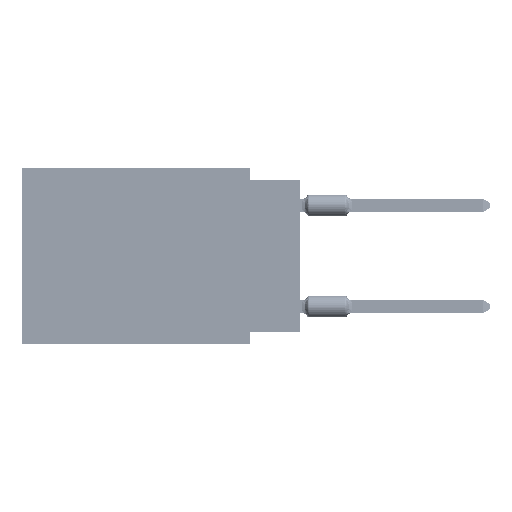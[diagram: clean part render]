
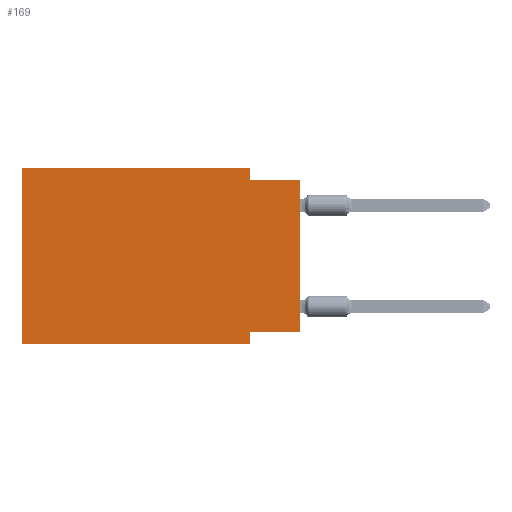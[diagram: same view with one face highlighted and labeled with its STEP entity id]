
A CAD part, left-side view. The second image highlights one B-rep face of the part: STEP entity #169.
In plain terms, the highlighted planar face has unit normal (-1, 0, 0).
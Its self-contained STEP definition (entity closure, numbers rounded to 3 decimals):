
#169 = ADVANCED_FACE ( 'NONE', ( #64927 ), #10518, .F. ) ;
#2532 = LINE ( 'NONE', #24767, #67308 ) ;
#3921 = LINE ( 'NONE', #25838, #35706 ) ;
#4976 = EDGE_CURVE ( 'NONE', #27019, #26516, #2532, .T. ) ;
#5753 = DIRECTION ( 'NONE',  ( 0., 0., -1. ) ) ;
#5892 = VECTOR ( 'NONE', #63146, 1000. ) ;
#6771 = ORIENTED_EDGE ( 'NONE', *, *, #37683, .F. ) ;
#7550 = DIRECTION ( 'NONE',  ( 0., 0., 1. ) ) ;
#10518 = PLANE ( 'NONE',  #65949 ) ;
#13570 = ORIENTED_EDGE ( 'NONE', *, *, #66424, .F. ) ;
#14536 = DIRECTION ( 'NONE',  ( 0., -1., 0. ) ) ;
#15593 = DIRECTION ( 'NONE',  ( 0., 0., -1. ) ) ;
#16460 = EDGE_LOOP ( 'NONE', ( #61674, #40314, #13570, #62673, #17269, #16903, #51655, #6771 ) ) ;
#16903 = ORIENTED_EDGE ( 'NONE', *, *, #4976, .T. ) ;
#17269 = ORIENTED_EDGE ( 'NONE', *, *, #38700, .F. ) ;
#18511 = CARTESIAN_POINT ( 'NONE',  ( 0., 0., -0.635 ) ) ;
#19266 = CARTESIAN_POINT ( 'NONE',  ( 0., 2.54, -8.89 ) ) ;
#19798 = CARTESIAN_POINT ( 'NONE',  ( 0., 13.97, 0. ) ) ;
#20078 = VECTOR ( 'NONE', #61257, 1000. ) ;
#20486 = DIRECTION ( 'NONE',  ( 0., 0., -1. ) ) ;
#23915 = VERTEX_POINT ( 'NONE', #41439 ) ;
#24767 = CARTESIAN_POINT ( 'NONE',  ( 0., 13.97, -8.89 ) ) ;
#25838 = CARTESIAN_POINT ( 'NONE',  ( 0., 2.54, -8.89 ) ) ;
#26011 = LINE ( 'NONE', #65151, #56744 ) ;
#26516 = VERTEX_POINT ( 'NONE', #19266 ) ;
#27019 = VERTEX_POINT ( 'NONE', #66199 ) ;
#29850 = LINE ( 'NONE', #41194, #5892 ) ;
#29943 = VERTEX_POINT ( 'NONE', #40937 ) ;
#30216 = LINE ( 'NONE', #57983, #48218 ) ;
#32770 = CARTESIAN_POINT ( 'NONE',  ( 0., 13.97, 0. ) ) ;
#33168 = VERTEX_POINT ( 'NONE', #66896 ) ;
#35706 = VECTOR ( 'NONE', #15593, 1000. ) ;
#37683 = EDGE_CURVE ( 'NONE', #29943, #44548, #29850, .T. ) ;
#38700 = EDGE_CURVE ( 'NONE', #27019, #33168, #26011, .T. ) ;
#40314 = ORIENTED_EDGE ( 'NONE', *, *, #68638, .F. ) ;
#40388 = EDGE_CURVE ( 'NONE', #44548, #26516, #3921, .T. ) ;
#40937 = CARTESIAN_POINT ( 'NONE',  ( 0., 0., -8.255 ) ) ;
#41194 = CARTESIAN_POINT ( 'NONE',  ( 0., 0., -8.255 ) ) ;
#41439 = CARTESIAN_POINT ( 'NONE',  ( 0., 0., -0.635 ) ) ;
#44548 = VERTEX_POINT ( 'NONE', #60136 ) ;
#44883 = DIRECTION ( 'NONE',  ( 0., 0., 1. ) ) ;
#44993 = VERTEX_POINT ( 'NONE', #60790 ) ;
#48218 = VECTOR ( 'NONE', #7550, 1000. ) ;
#48435 = VERTEX_POINT ( 'NONE', #68672 ) ;
#50662 = LINE ( 'NONE', #18511, #20078 ) ;
#51655 = ORIENTED_EDGE ( 'NONE', *, *, #40388, .F. ) ;
#53031 = DIRECTION ( 'NONE',  ( 0., -1., 0. ) ) ;
#54819 = EDGE_CURVE ( 'NONE', #29943, #23915, #30216, .T. ) ;
#55788 = DIRECTION ( 'NONE',  ( 1., 0., 0. ) ) ;
#56744 = VECTOR ( 'NONE', #44883, 1000. ) ;
#57219 = EDGE_CURVE ( 'NONE', #33168, #44993, #57783, .T. ) ;
#57783 = LINE ( 'NONE', #19798, #71575 ) ;
#57983 = CARTESIAN_POINT ( 'NONE',  ( 0., 0., 0. ) ) ;
#58392 = VECTOR ( 'NONE', #20486, 1000. ) ;
#58544 = LINE ( 'NONE', #70557, #58392 ) ;
#60136 = CARTESIAN_POINT ( 'NONE',  ( 0., 2.54, -8.255 ) ) ;
#60790 = CARTESIAN_POINT ( 'NONE',  ( 0., 2.54, 0. ) ) ;
#61257 = DIRECTION ( 'NONE',  ( 0., -1., 0. ) ) ;
#61674 = ORIENTED_EDGE ( 'NONE', *, *, #54819, .T. ) ;
#62673 = ORIENTED_EDGE ( 'NONE', *, *, #57219, .F. ) ;
#63146 = DIRECTION ( 'NONE',  ( 0., 1., 0. ) ) ;
#64927 = FACE_OUTER_BOUND ( 'NONE', #16460, .T. ) ;
#65151 = CARTESIAN_POINT ( 'NONE',  ( 0., 13.97, 0. ) ) ;
#65949 = AXIS2_PLACEMENT_3D ( 'NONE', #32770, #55788, #5753 ) ;
#66199 = CARTESIAN_POINT ( 'NONE',  ( 0., 13.97, -8.89 ) ) ;
#66424 = EDGE_CURVE ( 'NONE', #44993, #48435, #58544, .T. ) ;
#66896 = CARTESIAN_POINT ( 'NONE',  ( 0., 13.97, 0. ) ) ;
#67308 = VECTOR ( 'NONE', #14536, 1000. ) ;
#68638 = EDGE_CURVE ( 'NONE', #48435, #23915, #50662, .T. ) ;
#68672 = CARTESIAN_POINT ( 'NONE',  ( 0., 2.54, -0.635 ) ) ;
#70557 = CARTESIAN_POINT ( 'NONE',  ( 0., 2.54, 0. ) ) ;
#71575 = VECTOR ( 'NONE', #53031, 1000. ) ;
